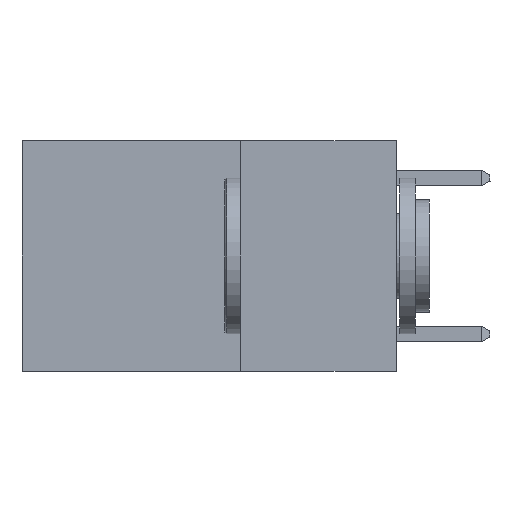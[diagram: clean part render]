
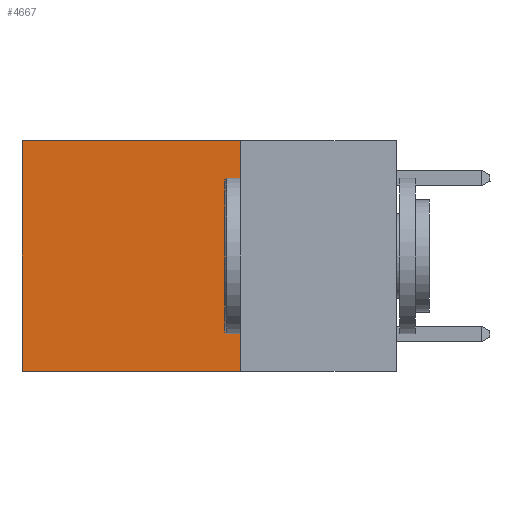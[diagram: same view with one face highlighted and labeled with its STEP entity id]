
A CAD part, left-side view. The second image highlights one B-rep face of the part: STEP entity #4667.
In plain terms, the highlighted planar face has unit normal (-1, 0, 0).
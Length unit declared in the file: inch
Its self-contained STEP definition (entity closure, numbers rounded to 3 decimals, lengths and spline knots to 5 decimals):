
#163 = CARTESIAN_POINT ( 'NONE',  ( 0.2625, 0.25, 0. ) ) ;
#436 = CARTESIAN_POINT ( 'NONE',  ( 0.2625, 0.25, -0.37 ) ) ;
#450 = EDGE_CURVE ( 'NONE', #2424, #2975, #3802, .T. ) ;
#733 = VERTEX_POINT ( 'NONE', #3177 ) ;
#819 = CARTESIAN_POINT ( 'NONE',  ( 0.2625, 0.25, 0. ) ) ;
#906 = VECTOR ( 'NONE', #7065, 39.37008 ) ;
#1043 = VECTOR ( 'NONE', #8924, 39.37008 ) ;
#1113 = CARTESIAN_POINT ( 'NONE',  ( 0.2625, 0.25, 0. ) ) ;
#1246 = LINE ( 'NONE', #436, #1043 ) ;
#2109 = AXIS2_PLACEMENT_3D ( 'NONE', #4713, #4798, #5489 ) ;
#2424 = VERTEX_POINT ( 'NONE', #6914 ) ;
#2543 = ORIENTED_EDGE ( 'NONE', *, *, #5176, .T. ) ;
#2647 = EDGE_CURVE ( 'NONE', #6825, #733, #5525, .T. ) ;
#2959 = VECTOR ( 'NONE', #5746, 39.37008 ) ;
#2975 = VERTEX_POINT ( 'NONE', #3607 ) ;
#3177 = CARTESIAN_POINT ( 'NONE',  ( 0.2625, 0.25, -0.37 ) ) ;
#3607 = CARTESIAN_POINT ( 'NONE',  ( 0.2625, 0.6, -0.37 ) ) ;
#3695 = ORIENTED_EDGE ( 'NONE', *, *, #2647, .F. ) ;
#3802 = LINE ( 'NONE', #6233, #4346 ) ;
#4346 = VECTOR ( 'NONE', #6937, 39.37008 ) ;
#4667 = ADVANCED_FACE ( 'NONE', ( #6647 ), #8265, .F. ) ;
#4713 = CARTESIAN_POINT ( 'NONE',  ( 0.2625, 0.25, 0. ) ) ;
#4798 = DIRECTION ( 'NONE',  ( 1., 0., 0. ) ) ;
#4831 = EDGE_CURVE ( 'NONE', #733, #2975, #1246, .T. ) ;
#4912 = EDGE_LOOP ( 'NONE', ( #6517, #6443, #3695, #2543 ) ) ;
#5176 = EDGE_CURVE ( 'NONE', #6825, #2424, #8059, .T. ) ;
#5489 = DIRECTION ( 'NONE',  ( 0., 0., -1. ) ) ;
#5525 = LINE ( 'NONE', #163, #906 ) ;
#5746 = DIRECTION ( 'NONE',  ( 0., 1., 0. ) ) ;
#6233 = CARTESIAN_POINT ( 'NONE',  ( 0.2625, 0.6, 0. ) ) ;
#6443 = ORIENTED_EDGE ( 'NONE', *, *, #4831, .F. ) ;
#6517 = ORIENTED_EDGE ( 'NONE', *, *, #450, .T. ) ;
#6647 = FACE_OUTER_BOUND ( 'NONE', #4912, .T. ) ;
#6825 = VERTEX_POINT ( 'NONE', #1113 ) ;
#6914 = CARTESIAN_POINT ( 'NONE',  ( 0.2625, 0.6, 0. ) ) ;
#6937 = DIRECTION ( 'NONE',  ( 0., 0., -1. ) ) ;
#7065 = DIRECTION ( 'NONE',  ( 0., 0., -1. ) ) ;
#8059 = LINE ( 'NONE', #819, #2959 ) ;
#8265 = PLANE ( 'NONE',  #2109 ) ;
#8924 = DIRECTION ( 'NONE',  ( 0., 1., 0. ) ) ;
